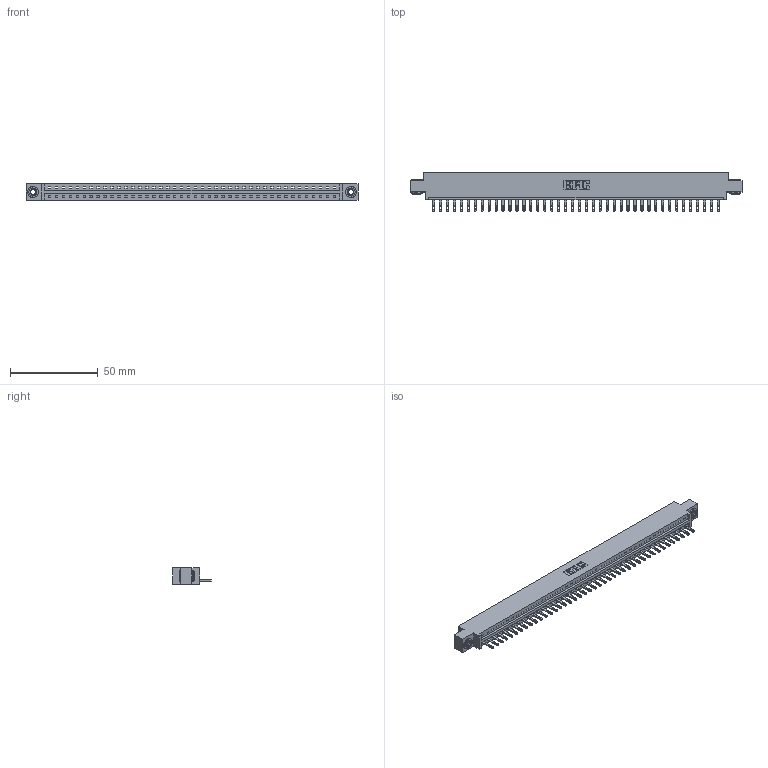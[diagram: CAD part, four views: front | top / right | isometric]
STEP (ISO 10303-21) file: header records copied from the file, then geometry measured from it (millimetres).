
FILE_DESCRIPTION (( 'STEP AP203' ), '1' );
FILE_NAME ('887-042-500-603.STEP', '2020-09-21T00:03:14', ( '' ), ( '' ), 'SwSTEP 2.0', 'SolidWorks 2020', '' );
FILE_SCHEMA (( 'CONFIG_CONTROL_DESIGN' ));
Length unit declared in the file: inch
Products named in the file (4): 345-292-001_345-293-100; 887-042-500-603; 837 Part_0.170 Offset - 0.156 Dia-TH; 345-250-002_345-250-002-102
Assembly tree (45 placements, depth 2):
  887-042-500-603
    837 Part_0.170 Offset - 0.156 Dia-TH
    345-292-001_345-293-100  x42
    345-250-002_345-250-002-102  x2
Bounding box: 189.43 x 21.85 x 9.4 mm (x, y, z)
Volume: 19616.3 mm3; surface area: 20697.7 mm2
Topology: 45 solids, 45 shells, 2592 faces, 7959 edges, 5302 vertices
Faces by surface type: plane 1764, cylinder 820, cone 8
Entity records: 31932 total; most frequent: CARTESIAN_POINT 5539, ORIENTED_EDGE 5510, DIRECTION 4697, EDGE_CURVE 2755, VECTOR 2599, LINE 2599, VERTEX_POINT 1834, AXIS2_PLACEMENT_3D 1049
